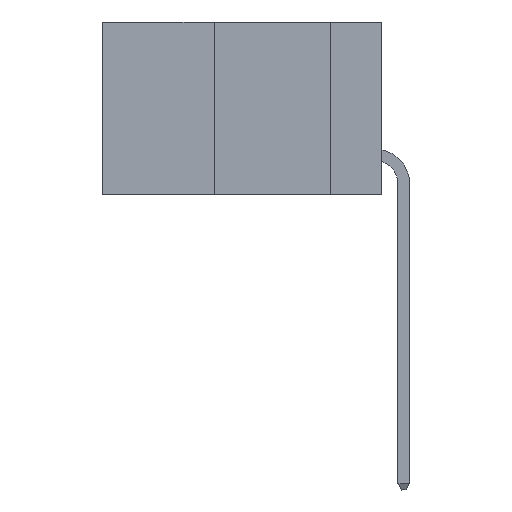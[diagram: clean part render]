
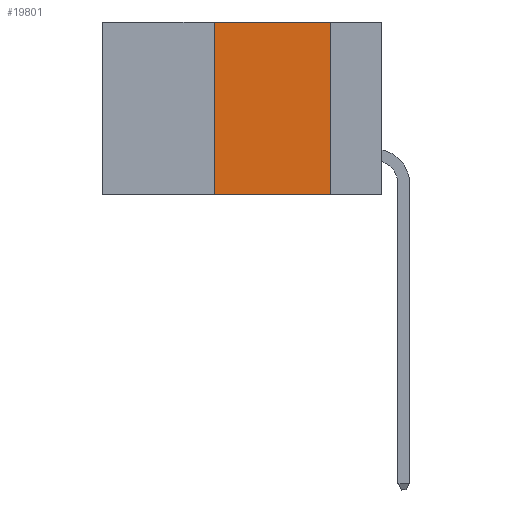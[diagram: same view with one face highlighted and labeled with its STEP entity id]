
A CAD part, left-side view. The second image highlights one B-rep face of the part: STEP entity #19801.
In plain terms, the highlighted planar face has unit normal (-1, 0, 0).
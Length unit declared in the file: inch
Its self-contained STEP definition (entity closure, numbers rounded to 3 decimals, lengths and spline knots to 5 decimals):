
#1624 = DIRECTION ( 'NONE',  ( 0., 0., -1. ) ) ;
#2131 = LINE ( 'NONE', #24489, #17588 ) ;
#2609 = VERTEX_POINT ( 'NONE', #38056 ) ;
#3363 = VERTEX_POINT ( 'NONE', #29730 ) ;
#4791 = PLANE ( 'NONE',  #48126 ) ;
#5628 = EDGE_CURVE ( 'NONE', #22876, #2609, #2131, .T. ) ;
#5860 = EDGE_CURVE ( 'NONE', #3363, #2609, #22859, .T. ) ;
#8488 = EDGE_CURVE ( 'NONE', #3363, #34337, #14306, .T. ) ;
#8789 = CARTESIAN_POINT ( 'NONE',  ( 0., 0.36, 0. ) ) ;
#9179 = LINE ( 'NONE', #15005, #10369 ) ;
#9766 = FACE_OUTER_BOUND ( 'NONE', #46149, .T. ) ;
#10369 = VECTOR ( 'NONE', #15651, 39.37008 ) ;
#12593 = DIRECTION ( 'NONE',  ( 0., 0., 1. ) ) ;
#14306 = LINE ( 'NONE', #8789, #17865 ) ;
#14581 = VECTOR ( 'NONE', #21874, 39.37008 ) ;
#15005 = CARTESIAN_POINT ( 'NONE',  ( 0., 0.6, 0. ) ) ;
#15651 = DIRECTION ( 'NONE',  ( 0., -1., 0. ) ) ;
#17588 = VECTOR ( 'NONE', #1624, 39.37008 ) ;
#17865 = VECTOR ( 'NONE', #12593, 39.37008 ) ;
#18248 = CARTESIAN_POINT ( 'NONE',  ( 0., 0.6, -0.37 ) ) ;
#19113 = EDGE_CURVE ( 'NONE', #34337, #22876, #9179, .T. ) ;
#19801 = ADVANCED_FACE ( 'NONE', ( #9766 ), #4791, .F. ) ;
#21209 = ORIENTED_EDGE ( 'NONE', *, *, #19113, .F. ) ;
#21874 = DIRECTION ( 'NONE',  ( 0., -1., 0. ) ) ;
#22859 = LINE ( 'NONE', #18248, #14581 ) ;
#22876 = VERTEX_POINT ( 'NONE', #34137 ) ;
#24489 = CARTESIAN_POINT ( 'NONE',  ( 0., 0.11, 0. ) ) ;
#27928 = CARTESIAN_POINT ( 'NONE',  ( 0., 0.36, 0. ) ) ;
#29730 = CARTESIAN_POINT ( 'NONE',  ( 0., 0.36, -0.37 ) ) ;
#31762 = ORIENTED_EDGE ( 'NONE', *, *, #8488, .F. ) ;
#34137 = CARTESIAN_POINT ( 'NONE',  ( 0., 0.11, 0. ) ) ;
#34337 = VERTEX_POINT ( 'NONE', #27928 ) ;
#38056 = CARTESIAN_POINT ( 'NONE',  ( 0., 0.11, -0.37 ) ) ;
#42537 = DIRECTION ( 'NONE',  ( 0., 0., -1. ) ) ;
#42691 = CARTESIAN_POINT ( 'NONE',  ( 0., 0.6, 0. ) ) ;
#42735 = ORIENTED_EDGE ( 'NONE', *, *, #5860, .T. ) ;
#46149 = EDGE_LOOP ( 'NONE', ( #46558, #21209, #31762, #42735 ) ) ;
#46558 = ORIENTED_EDGE ( 'NONE', *, *, #5628, .F. ) ;
#46984 = DIRECTION ( 'NONE',  ( 1., 0., 0. ) ) ;
#48126 = AXIS2_PLACEMENT_3D ( 'NONE', #42691, #46984, #42537 ) ;
